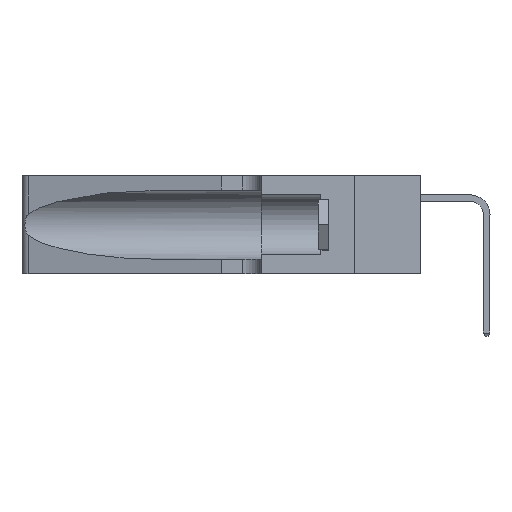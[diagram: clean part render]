
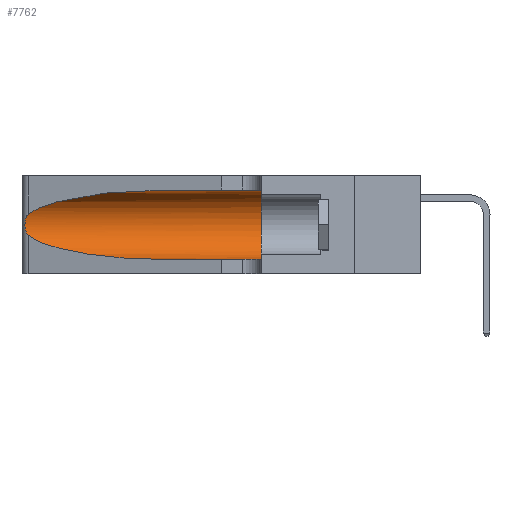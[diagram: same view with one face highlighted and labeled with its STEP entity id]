
A CAD part, left-side view. The second image highlights one B-rep face of the part: STEP entity #7762.
In plain terms, the highlighted cylindrical face has radius 3.308 mm (diameter 6.617 mm), a partial arc.
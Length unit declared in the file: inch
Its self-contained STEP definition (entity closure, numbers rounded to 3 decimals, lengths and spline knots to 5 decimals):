
#354 = CARTESIAN_POINT ( 'NONE',  ( 0.1305, 0.35, 0.31525 ) ) ;
#418 = ORIENTED_EDGE ( 'NONE', *, *, #3282, .T. ) ;
#670 =( BOUNDED_CURVE ( )  B_SPLINE_CURVE ( 3, ( #6019, #14247, #10152, #1917 ),
 .UNSPECIFIED., .F., .F. ) 
 B_SPLINE_CURVE_WITH_KNOTS ( ( 4, 4 ),
 ( 3.44316, 4.71239 ),
 .UNSPECIFIED. ) 
 CURVE ( )  GEOMETRIC_REPRESENTATION_ITEM ( )  RATIONAL_B_SPLINE_CURVE ( ( 1., 0.87, 0.87, 1. ) ) 
 REPRESENTATION_ITEM ( '' )  );
#682 = CARTESIAN_POINT ( 'NONE',  ( 0.1305, 0.35, 0.05475 ) ) ;
#736 = CARTESIAN_POINT ( 'NONE',  ( 0.25555, 1.22994, 0.2215 ) ) ;
#804 = CARTESIAN_POINT ( 'NONE',  ( 0.25555, 1.22993, 0.14849 ) ) ;
#923 = DIRECTION ( 'NONE',  ( 0., 0., 1. ) ) ;
#1307 = FACE_OUTER_BOUND ( 'NONE', #17797, .T. ) ;
#1829 = CARTESIAN_POINT ( 'NONE',  ( 0.1305, 0.72297, 0.31525 ) ) ;
#1917 = CARTESIAN_POINT ( 'NONE',  ( 0.1305, 0.72297, 0.05475 ) ) ;
#1978 = CARTESIAN_POINT ( 'NONE',  ( 0.25487, 1.22718, 0.14631 ) ) ;
#2057 = DIRECTION ( 'NONE',  ( 0., -1., 0. ) ) ;
#2528 = VECTOR ( 'NONE', #2057, 39.37008 ) ;
#3282 = EDGE_CURVE ( 'NONE', #15821, #13550, #6192, .T. ) ;
#3515 = CARTESIAN_POINT ( 'NONE',  ( 0.25787, 1.23484, 0.2124 ) ) ;
#3752 = EDGE_CURVE ( 'NONE', #17608, #10910, #9823, .T. ) ;
#3818 = ORIENTED_EDGE ( 'NONE', *, *, #7514, .T. ) ;
#3822 = VERTEX_POINT ( 'NONE', #12793 ) ;
#3896 = VERTEX_POINT ( 'NONE', #1978 ) ;
#4919 = CARTESIAN_POINT ( 'NONE',  ( 0.26018, 1.23835, 0.19895 ) ) ;
#5200 = ORIENTED_EDGE ( 'NONE', *, *, #3752, .F. ) ;
#5250 = ORIENTED_EDGE ( 'NONE', *, *, #10313, .F. ) ;
#5985 = CARTESIAN_POINT ( 'NONE',  ( 0.2373, 1.15595, 0.28018 ) ) ;
#6019 = CARTESIAN_POINT ( 'NONE',  ( 0.25487, 1.22718, 0.14631 ) ) ;
#6192 = LINE ( 'NONE', #11650, #2528 ) ;
#6227 = CARTESIAN_POINT ( 'NONE',  ( 0.25487, 1.22718, 0.22369 ) ) ;
#6248 = DIRECTION ( 'NONE',  ( 0., -1., 0. ) ) ;
#6282 = CARTESIAN_POINT ( 'NONE',  ( 0.26075, 1.23896, 0.178 ) ) ;
#6485 = EDGE_CURVE ( 'NONE', #3822, #3896, #7054, .T. ) ;
#7054 = B_SPLINE_CURVE_WITH_KNOTS ( 'NONE', 3,
 ( #6227, #736, #11718, #3515, #13137, #4919, #14508, #6282, #15868, #7646, #17243, #9022, #804, #10414 ),
 .UNSPECIFIED., .F., .F.,
 ( 4, 2, 2, 2, 2, 2, 4 ),
 ( 0., 0.00027, 0.00053, 0.00107, 0.0016, 0.00187, 0.00214 ),
 .UNSPECIFIED. ) ;
#7140 = DIRECTION ( 'NONE',  ( 0., -1., 0. ) ) ;
#7514 = EDGE_CURVE ( 'NONE', #3896, #15821, #670, .T. ) ;
#7614 = DIRECTION ( 'NONE',  ( 0., 0., -1. ) ) ;
#7646 = CARTESIAN_POINT ( 'NONE',  ( 0.25856, 1.23593, 0.16098 ) ) ;
#7762 = ADVANCED_FACE ( 'NONE', ( #1307 ), #11398, .F. ) ;
#7781 = AXIS2_PLACEMENT_3D ( 'NONE', #17364, #9153, #923 ) ;
#8795 = EDGE_CURVE ( 'NONE', #17608, #3822, #15315, .T. ) ;
#9022 = CARTESIAN_POINT ( 'NONE',  ( 0.25639, 1.23186, 0.15144 ) ) ;
#9153 = DIRECTION ( 'NONE',  ( 0., 1., 0. ) ) ;
#9823 = LINE ( 'NONE', #12669, #13054 ) ;
#10039 = AXIS2_PLACEMENT_3D ( 'NONE', #13105, #6248, #7614 ) ;
#10152 = CARTESIAN_POINT ( 'NONE',  ( 0.18966, 0.96281, 0.05475 ) ) ;
#10313 = EDGE_CURVE ( 'NONE', #10910, #13550, #14916, .T. ) ;
#10414 = CARTESIAN_POINT ( 'NONE',  ( 0.25487, 1.22718, 0.14631 ) ) ;
#10910 = VERTEX_POINT ( 'NONE', #354 ) ;
#11161 = ORIENTED_EDGE ( 'NONE', *, *, #6485, .T. ) ;
#11398 = CYLINDRICAL_SURFACE ( 'NONE', #10039, 0.13025 ) ;
#11428 = CARTESIAN_POINT ( 'NONE',  ( 0.18966, 0.96281, 0.31525 ) ) ;
#11650 = CARTESIAN_POINT ( 'NONE',  ( 0.1305, 1.61858, 0.05475 ) ) ;
#11718 = CARTESIAN_POINT ( 'NONE',  ( 0.25639, 1.23184, 0.21858 ) ) ;
#12669 = CARTESIAN_POINT ( 'NONE',  ( 0.1305, 1.61858, 0.31525 ) ) ;
#12793 = CARTESIAN_POINT ( 'NONE',  ( 0.25487, 1.22718, 0.22369 ) ) ;
#13054 = VECTOR ( 'NONE', #7140, 39.37008 ) ;
#13105 = CARTESIAN_POINT ( 'NONE',  ( 0.1305, 1.61858, 0.185 ) ) ;
#13137 = CARTESIAN_POINT ( 'NONE',  ( 0.25854, 1.2359, 0.20912 ) ) ;
#13550 = VERTEX_POINT ( 'NONE', #682 ) ;
#13595 = ORIENTED_EDGE ( 'NONE', *, *, #8795, .T. ) ;
#13942 = CARTESIAN_POINT ( 'NONE',  ( 0.1305, 0.72297, 0.31525 ) ) ;
#14247 = CARTESIAN_POINT ( 'NONE',  ( 0.2373, 1.15595, 0.08982 ) ) ;
#14508 = CARTESIAN_POINT ( 'NONE',  ( 0.26075, 1.23896, 0.19203 ) ) ;
#14916 = CIRCLE ( 'NONE', #7781, 0.13025 ) ;
#15315 =( BOUNDED_CURVE ( )  B_SPLINE_CURVE ( 3, ( #1829, #11428, #5985, #15576 ),
 .UNSPECIFIED., .F., .T. ) 
 B_SPLINE_CURVE_WITH_KNOTS ( ( 4, 4 ),
 ( 1.5708, 2.84003 ),
 .UNSPECIFIED. ) 
 CURVE ( )  GEOMETRIC_REPRESENTATION_ITEM ( )  RATIONAL_B_SPLINE_CURVE ( ( 1., 0.87, 0.87, 1. ) ) 
 REPRESENTATION_ITEM ( '' )  );
#15387 = CARTESIAN_POINT ( 'NONE',  ( 0.1305, 0.72297, 0.05475 ) ) ;
#15576 = CARTESIAN_POINT ( 'NONE',  ( 0.25487, 1.22718, 0.22369 ) ) ;
#15821 = VERTEX_POINT ( 'NONE', #15387 ) ;
#15868 = CARTESIAN_POINT ( 'NONE',  ( 0.26017, 1.23833, 0.17102 ) ) ;
#17243 = CARTESIAN_POINT ( 'NONE',  ( 0.25789, 1.23486, 0.15765 ) ) ;
#17364 = CARTESIAN_POINT ( 'NONE',  ( 0.1305, 0.35, 0.185 ) ) ;
#17608 = VERTEX_POINT ( 'NONE', #13942 ) ;
#17797 = EDGE_LOOP ( 'NONE', ( #13595, #11161, #3818, #418, #5250, #5200 ) ) ;
